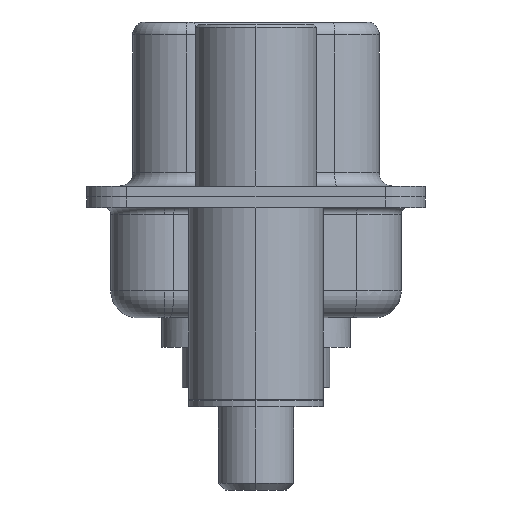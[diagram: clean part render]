
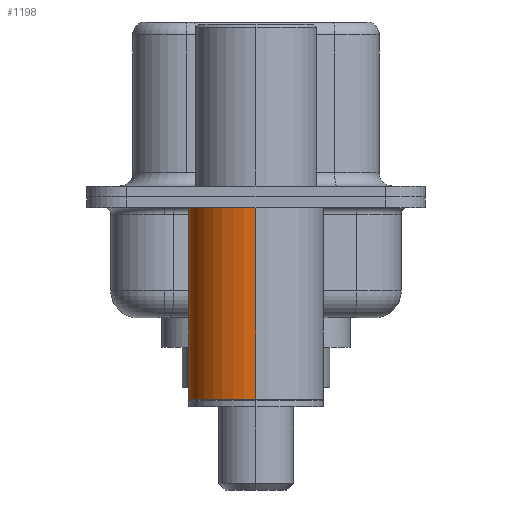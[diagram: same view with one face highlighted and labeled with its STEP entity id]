
A CAD part, left-side view. The second image highlights one B-rep face of the part: STEP entity #1198.
In plain terms, the highlighted cylindrical face has radius 2.5 mm (diameter 5 mm), a partial arc.
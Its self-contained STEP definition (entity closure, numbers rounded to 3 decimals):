
#905 = VERTEX_POINT ( 'NONE', #5410 ) ;
#975 = CARTESIAN_POINT ( 'NONE',  ( 2.5, 0., -0.4 ) ) ;
#1198 = ADVANCED_FACE ( 'NONE', ( #16958 ), #3074, .T. ) ;
#1206 = CARTESIAN_POINT ( 'NONE',  ( -2.5, 0., 0.581 ) ) ;
#1450 = EDGE_LOOP ( 'NONE', ( #21145, #8084, #21438, #1784 ) ) ;
#1784 = ORIENTED_EDGE ( 'NONE', *, *, #14889, .F. ) ;
#2728 = DIRECTION ( 'NONE',  ( 0., 0., 1. ) ) ;
#2799 = DIRECTION ( 'NONE',  ( 0., 0., 1. ) ) ;
#3074 = CYLINDRICAL_SURFACE ( 'NONE', #20466, 2.5 ) ;
#4662 = EDGE_CURVE ( 'NONE', #7063, #905, #17423, .T. ) ;
#4786 = EDGE_CURVE ( 'NONE', #18559, #905, #15245, .T. ) ;
#5410 = CARTESIAN_POINT ( 'NONE',  ( -2.5, 0., -0.4 ) ) ;
#5927 = VECTOR ( 'NONE', #2728, 1000. ) ;
#6932 = AXIS2_PLACEMENT_3D ( 'NONE', #10241, #2799, #13895 ) ;
#7063 = VERTEX_POINT ( 'NONE', #12750 ) ;
#7492 = CARTESIAN_POINT ( 'NONE',  ( 0., 0., 0.581 ) ) ;
#8084 = ORIENTED_EDGE ( 'NONE', *, *, #4662, .T. ) ;
#9418 = DIRECTION ( 'NONE',  ( 0., 0., 1. ) ) ;
#9674 = CARTESIAN_POINT ( 'NONE',  ( 2.5, 0., 0.581 ) ) ;
#10241 = CARTESIAN_POINT ( 'NONE',  ( 0., 0., -0.4 ) ) ;
#10250 = DIRECTION ( 'NONE',  ( 0., 0., 1. ) ) ;
#10775 = CARTESIAN_POINT ( 'NONE',  ( 2.5, 0., -7.525 ) ) ;
#12281 = VECTOR ( 'NONE', #14998, 1000. ) ;
#12313 = DIRECTION ( 'NONE',  ( 1., 0., 0. ) ) ;
#12750 = CARTESIAN_POINT ( 'NONE',  ( -2.5, 0., -7.525 ) ) ;
#13835 = CIRCLE ( 'NONE', #22245, 2.5 ) ;
#13895 = DIRECTION ( 'NONE',  ( 1., 0., 0. ) ) ;
#14889 = EDGE_CURVE ( 'NONE', #19022, #18559, #15180, .T. ) ;
#14998 = DIRECTION ( 'NONE',  ( 0., 0., 1. ) ) ;
#15180 = LINE ( 'NONE', #9674, #5927 ) ;
#15245 = CIRCLE ( 'NONE', #6932, 2.5 ) ;
#15717 = EDGE_CURVE ( 'NONE', #19022, #7063, #13835, .T. ) ;
#16958 = FACE_OUTER_BOUND ( 'NONE', #1450, .T. ) ;
#17423 = LINE ( 'NONE', #1206, #12281 ) ;
#18559 = VERTEX_POINT ( 'NONE', #975 ) ;
#19022 = VERTEX_POINT ( 'NONE', #10775 ) ;
#19843 = CARTESIAN_POINT ( 'NONE',  ( 0., 0., -7.525 ) ) ;
#20466 = AXIS2_PLACEMENT_3D ( 'NONE', #7492, #10250, #12313 ) ;
#21145 = ORIENTED_EDGE ( 'NONE', *, *, #15717, .T. ) ;
#21438 = ORIENTED_EDGE ( 'NONE', *, *, #4786, .F. ) ;
#21622 = DIRECTION ( 'NONE',  ( 1., 0., 0. ) ) ;
#22245 = AXIS2_PLACEMENT_3D ( 'NONE', #19843, #9418, #21622 ) ;
